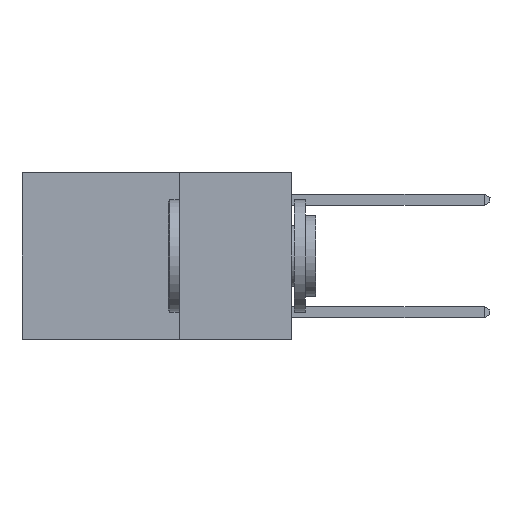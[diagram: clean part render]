
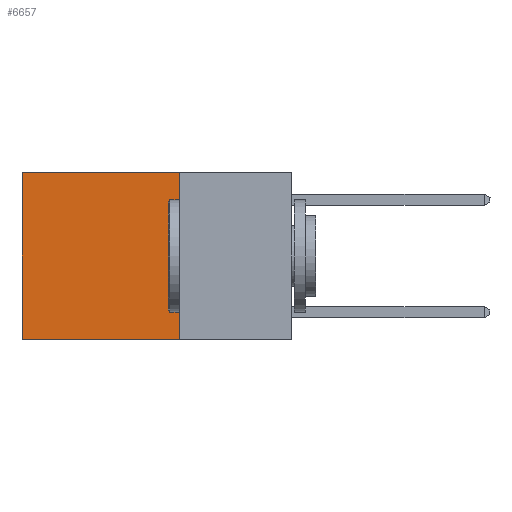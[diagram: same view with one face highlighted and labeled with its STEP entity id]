
A CAD part, left-side view. The second image highlights one B-rep face of the part: STEP entity #6657.
In plain terms, the highlighted planar face has unit normal (-1, 0, 0).
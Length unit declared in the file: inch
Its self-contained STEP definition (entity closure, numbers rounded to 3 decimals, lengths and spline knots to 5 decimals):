
#110 = EDGE_CURVE ( 'NONE', #19759, #7077, #15030, .T. ) ;
#571 = CARTESIAN_POINT ( 'NONE',  ( 0.2625, 0.25, 0. ) ) ;
#601 = CARTESIAN_POINT ( 'NONE',  ( 0.2625, 0.25, 0. ) ) ;
#2216 = DIRECTION ( 'NONE',  ( 1., 0., 0. ) ) ;
#2496 = CARTESIAN_POINT ( 'NONE',  ( 0.2625, 0.25, 0. ) ) ;
#2499 = LINE ( 'NONE', #10814, #6999 ) ;
#4131 = DIRECTION ( 'NONE',  ( 0., 1., 0. ) ) ;
#4703 = EDGE_LOOP ( 'NONE', ( #14658, #6779, #9598, #9492 ) ) ;
#6397 = CARTESIAN_POINT ( 'NONE',  ( 0.2625, 0.6, 0. ) ) ;
#6657 = ADVANCED_FACE ( 'NONE', ( #8690 ), #16943, .F. ) ;
#6703 = LINE ( 'NONE', #571, #17129 ) ;
#6779 = ORIENTED_EDGE ( 'NONE', *, *, #11253, .F. ) ;
#6999 = VECTOR ( 'NONE', #4131, 39.37008 ) ;
#7077 = VERTEX_POINT ( 'NONE', #12656 ) ;
#7092 = VECTOR ( 'NONE', #15895, 39.37008 ) ;
#7834 = CARTESIAN_POINT ( 'NONE',  ( 0.2625, 0.6, 0. ) ) ;
#8690 = FACE_OUTER_BOUND ( 'NONE', #4703, .T. ) ;
#9492 = ORIENTED_EDGE ( 'NONE', *, *, #16210, .T. ) ;
#9598 = ORIENTED_EDGE ( 'NONE', *, *, #19019, .F. ) ;
#10102 = DIRECTION ( 'NONE',  ( 0., 0., -1. ) ) ;
#10814 = CARTESIAN_POINT ( 'NONE',  ( 0.2625, 0.25, -0.37 ) ) ;
#11253 = EDGE_CURVE ( 'NONE', #11292, #7077, #2499, .T. ) ;
#11292 = VERTEX_POINT ( 'NONE', #17018 ) ;
#12619 = LINE ( 'NONE', #17285, #7092 ) ;
#12656 = CARTESIAN_POINT ( 'NONE',  ( 0.2625, 0.6, -0.37 ) ) ;
#13226 = DIRECTION ( 'NONE',  ( 0., 0., -1. ) ) ;
#13293 = VECTOR ( 'NONE', #13226, 39.37008 ) ;
#13437 = AXIS2_PLACEMENT_3D ( 'NONE', #601, #2216, #10102 ) ;
#14658 = ORIENTED_EDGE ( 'NONE', *, *, #110, .T. ) ;
#15030 = LINE ( 'NONE', #6397, #13293 ) ;
#15895 = DIRECTION ( 'NONE',  ( 0., 1., 0. ) ) ;
#16210 = EDGE_CURVE ( 'NONE', #19192, #19759, #12619, .T. ) ;
#16943 = PLANE ( 'NONE',  #13437 ) ;
#17018 = CARTESIAN_POINT ( 'NONE',  ( 0.2625, 0.25, -0.37 ) ) ;
#17129 = VECTOR ( 'NONE', #19850, 39.37008 ) ;
#17285 = CARTESIAN_POINT ( 'NONE',  ( 0.2625, 0.25, 0. ) ) ;
#19019 = EDGE_CURVE ( 'NONE', #19192, #11292, #6703, .T. ) ;
#19192 = VERTEX_POINT ( 'NONE', #2496 ) ;
#19759 = VERTEX_POINT ( 'NONE', #7834 ) ;
#19850 = DIRECTION ( 'NONE',  ( 0., 0., -1. ) ) ;
